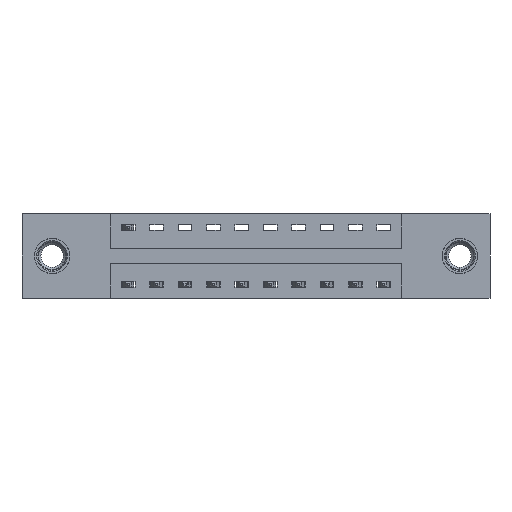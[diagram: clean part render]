
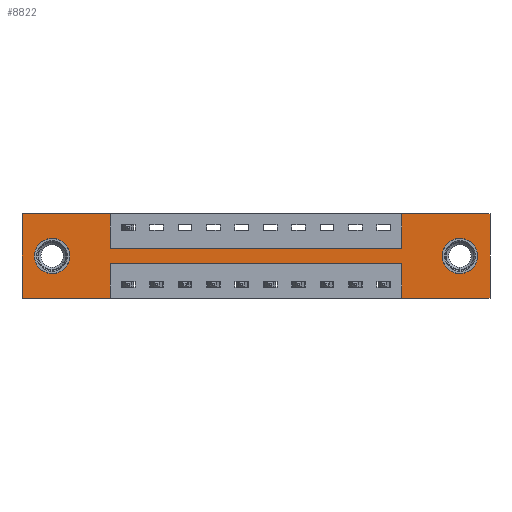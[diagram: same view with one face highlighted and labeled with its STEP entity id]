
A CAD part, front view. The second image highlights one B-rep face of the part: STEP entity #8822.
In plain terms, the highlighted planar face has unit normal (0, -1, 0).
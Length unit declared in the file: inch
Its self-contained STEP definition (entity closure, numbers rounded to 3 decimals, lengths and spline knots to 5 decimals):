
#252 = DIRECTION ( 'NONE',  ( 1., 0., 0. ) ) ;
#266 = VECTOR ( 'NONE', #3490, 39.37008 ) ;
#340 = AXIS2_PLACEMENT_3D ( 'NONE', #9653, #4228, #10537 ) ;
#367 = EDGE_CURVE ( 'NONE', #6139, #8540, #7498, .T. ) ;
#374 = LINE ( 'NONE', #8942, #7328 ) ;
#903 = CARTESIAN_POINT ( 'NONE',  ( 0., 0., 0. ) ) ;
#972 = CARTESIAN_POINT ( 'NONE',  ( 1.9275, 0., -0.185 ) ) ;
#976 = DIRECTION ( 'NONE',  ( -1., 0., 0. ) ) ;
#1192 = CARTESIAN_POINT ( 'NONE',  ( 1.9275, 0., -0.107 ) ) ;
#1198 = CARTESIAN_POINT ( 'NONE',  ( 1.6725, 0., -0.22 ) ) ;
#1221 = LINE ( 'NONE', #7119, #10551 ) ;
#1302 = CARTESIAN_POINT ( 'NONE',  ( 0., 0., 0. ) ) ;
#1346 = EDGE_CURVE ( 'NONE', #4024, #10152, #8497, .T. ) ;
#1392 = ORIENTED_EDGE ( 'NONE', *, *, #9641, .T. ) ;
#1459 = DIRECTION ( 'NONE',  ( -1., 0., 0. ) ) ;
#1496 = VECTOR ( 'NONE', #4390, 39.37008 ) ;
#1803 = ORIENTED_EDGE ( 'NONE', *, *, #7420, .T. ) ;
#1823 = EDGE_CURVE ( 'NONE', #10026, #1853, #6483, .T. ) ;
#1853 = VERTEX_POINT ( 'NONE', #1192 ) ;
#1889 = DIRECTION ( 'NONE',  ( 0., 0., -1. ) ) ;
#2069 = CARTESIAN_POINT ( 'NONE',  ( 1.9275, 0., -0.185 ) ) ;
#2090 = CARTESIAN_POINT ( 'NONE',  ( 1.6725, 0., -0.37 ) ) ;
#2194 = EDGE_LOOP ( 'NONE', ( #1803, #1392 ) ) ;
#2196 = DIRECTION ( 'NONE',  ( 1., 0., 0. ) ) ;
#2209 = PLANE ( 'NONE',  #7696 ) ;
#2290 = VECTOR ( 'NONE', #5743, 39.37008 ) ;
#2318 = LINE ( 'NONE', #3157, #11659 ) ;
#2573 = CARTESIAN_POINT ( 'NONE',  ( 0.3875, 0., 0. ) ) ;
#2576 = LINE ( 'NONE', #2090, #2290 ) ;
#2619 = DIRECTION ( 'NONE',  ( 0., 0., 1. ) ) ;
#2634 = ORIENTED_EDGE ( 'NONE', *, *, #9191, .T. ) ;
#2656 = ORIENTED_EDGE ( 'NONE', *, *, #367, .F. ) ;
#2724 = VECTOR ( 'NONE', #976, 39.37008 ) ;
#2778 = ORIENTED_EDGE ( 'NONE', *, *, #4403, .F. ) ;
#2842 = DIRECTION ( 'NONE',  ( 0., 1., 0. ) ) ;
#2978 = DIRECTION ( 'NONE',  ( 0., 0., -1. ) ) ;
#3028 = EDGE_LOOP ( 'NONE', ( #2634, #3465 ) ) ;
#3130 = DIRECTION ( 'NONE',  ( 0., -1., 0. ) ) ;
#3157 = CARTESIAN_POINT ( 'NONE',  ( 0., 0., -0.37 ) ) ;
#3262 = CARTESIAN_POINT ( 'NONE',  ( 1.6725, 0., -0.37 ) ) ;
#3268 = EDGE_CURVE ( 'NONE', #8540, #5853, #4088, .T. ) ;
#3384 = FACE_BOUND ( 'NONE', #2194, .T. ) ;
#3427 = CIRCLE ( 'NONE', #11123, 0.078 ) ;
#3465 = ORIENTED_EDGE ( 'NONE', *, *, #1823, .T. ) ;
#3490 = DIRECTION ( 'NONE',  ( 0., 0., -1. ) ) ;
#3493 = DIRECTION ( 'NONE',  ( 0., 0., 1. ) ) ;
#3627 = ORIENTED_EDGE ( 'NONE', *, *, #6941, .F. ) ;
#3734 = LINE ( 'NONE', #6914, #8263 ) ;
#3887 = LINE ( 'NONE', #9819, #1496 ) ;
#3912 = ORIENTED_EDGE ( 'NONE', *, *, #7568, .F. ) ;
#3925 = DIRECTION ( 'NONE',  ( 1., 0., 0. ) ) ;
#3987 = VERTEX_POINT ( 'NONE', #1198 ) ;
#4024 = VERTEX_POINT ( 'NONE', #7601 ) ;
#4077 = ORIENTED_EDGE ( 'NONE', *, *, #1346, .F. ) ;
#4088 = LINE ( 'NONE', #11111, #10723 ) ;
#4228 = DIRECTION ( 'NONE',  ( 0., 1., 0. ) ) ;
#4321 = VERTEX_POINT ( 'NONE', #7963 ) ;
#4349 = ORIENTED_EDGE ( 'NONE', *, *, #7541, .F. ) ;
#4390 = DIRECTION ( 'NONE',  ( 0., 0., -1. ) ) ;
#4403 = EDGE_CURVE ( 'NONE', #5853, #4321, #1221, .T. ) ;
#4492 = VERTEX_POINT ( 'NONE', #903 ) ;
#4601 = ORIENTED_EDGE ( 'NONE', *, *, #11670, .F. ) ;
#4833 = CIRCLE ( 'NONE', #7230, 0.078 ) ;
#5074 = AXIS2_PLACEMENT_3D ( 'NONE', #2069, #8426, #2978 ) ;
#5113 = LINE ( 'NONE', #6392, #2724 ) ;
#5253 = EDGE_CURVE ( 'NONE', #5287, #4024, #3887, .T. ) ;
#5287 = VERTEX_POINT ( 'NONE', #8041 ) ;
#5443 = CARTESIAN_POINT ( 'NONE',  ( 0.3875, 0., -0.15 ) ) ;
#5524 = CARTESIAN_POINT ( 'NONE',  ( 0.1325, 0., -0.263 ) ) ;
#5576 = CARTESIAN_POINT ( 'NONE',  ( 0.3875, 0., 0. ) ) ;
#5631 = EDGE_CURVE ( 'NONE', #10966, #6273, #2318, .T. ) ;
#5743 = DIRECTION ( 'NONE',  ( 0., 0., 1. ) ) ;
#5853 = VERTEX_POINT ( 'NONE', #7983 ) ;
#5865 = DIRECTION ( 'NONE',  ( -1., 0., 0. ) ) ;
#6052 = VECTOR ( 'NONE', #1459, 39.37008 ) ;
#6139 = VERTEX_POINT ( 'NONE', #5576 ) ;
#6273 = VERTEX_POINT ( 'NONE', #8519 ) ;
#6392 = CARTESIAN_POINT ( 'NONE',  ( 0.3875, 0., -0.22 ) ) ;
#6483 = CIRCLE ( 'NONE', #5074, 0.078 ) ;
#6914 = CARTESIAN_POINT ( 'NONE',  ( 0.3875, 0., -0.37 ) ) ;
#6941 = EDGE_CURVE ( 'NONE', #4321, #5287, #8425, .T. ) ;
#7119 = CARTESIAN_POINT ( 'NONE',  ( 1.6725, 0., 0. ) ) ;
#7153 = EDGE_CURVE ( 'NONE', #8580, #10966, #3734, .T. ) ;
#7196 = ORIENTED_EDGE ( 'NONE', *, *, #7401, .F. ) ;
#7230 = AXIS2_PLACEMENT_3D ( 'NONE', #8281, #2842, #9211 ) ;
#7307 = DIRECTION ( 'NONE',  ( 0., 1., 0. ) ) ;
#7328 = VECTOR ( 'NONE', #3493, 39.37008 ) ;
#7401 = EDGE_CURVE ( 'NONE', #3987, #8580, #5113, .T. ) ;
#7420 = EDGE_CURVE ( 'NONE', #8113, #10554, #4833, .T. ) ;
#7498 = LINE ( 'NONE', #2573, #266 ) ;
#7541 = EDGE_CURVE ( 'NONE', #10152, #3987, #2576, .T. ) ;
#7568 = EDGE_CURVE ( 'NONE', #4492, #6139, #9257, .T. ) ;
#7601 = CARTESIAN_POINT ( 'NONE',  ( 2.06, 0., -0.37 ) ) ;
#7696 = AXIS2_PLACEMENT_3D ( 'NONE', #8582, #3130, #9472 ) ;
#7728 = CARTESIAN_POINT ( 'NONE',  ( 0., 0., -0.37 ) ) ;
#7916 = FACE_OUTER_BOUND ( 'NONE', #8003, .T. ) ;
#7963 = CARTESIAN_POINT ( 'NONE',  ( 1.6725, 0., 0. ) ) ;
#7983 = CARTESIAN_POINT ( 'NONE',  ( 1.6725, 0., -0.15 ) ) ;
#8003 = EDGE_LOOP ( 'NONE', ( #9877, #7196, #4349, #4077, #8021, #3627, #2778, #9172, #2656, #3912, #4601, #11711 ) ) ;
#8021 = ORIENTED_EDGE ( 'NONE', *, *, #5253, .F. ) ;
#8041 = CARTESIAN_POINT ( 'NONE',  ( 2.06, 0., 0. ) ) ;
#8113 = VERTEX_POINT ( 'NONE', #9300 ) ;
#8263 = VECTOR ( 'NONE', #8701, 39.37008 ) ;
#8281 = CARTESIAN_POINT ( 'NONE',  ( 0.1325, 0., -0.185 ) ) ;
#8425 = LINE ( 'NONE', #11168, #10231 ) ;
#8426 = DIRECTION ( 'NONE',  ( 0., 1., 0. ) ) ;
#8497 = LINE ( 'NONE', #7728, #6052 ) ;
#8519 = CARTESIAN_POINT ( 'NONE',  ( 0., 0., -0.37 ) ) ;
#8540 = VERTEX_POINT ( 'NONE', #5443 ) ;
#8580 = VERTEX_POINT ( 'NONE', #10012 ) ;
#8582 = CARTESIAN_POINT ( 'NONE',  ( 0., 0., -0.37 ) ) ;
#8701 = DIRECTION ( 'NONE',  ( 0., 0., -1. ) ) ;
#8822 = ADVANCED_FACE ( 'NONE', ( #10311, #3384, #7916 ), #2209, .T. ) ;
#8942 = CARTESIAN_POINT ( 'NONE',  ( 0., 0., 0. ) ) ;
#9172 = ORIENTED_EDGE ( 'NONE', *, *, #3268, .F. ) ;
#9191 = EDGE_CURVE ( 'NONE', #1853, #10026, #3427, .T. ) ;
#9211 = DIRECTION ( 'NONE',  ( 0., 0., 1. ) ) ;
#9257 = LINE ( 'NONE', #1302, #11347 ) ;
#9300 = CARTESIAN_POINT ( 'NONE',  ( 0.1325, 0., -0.107 ) ) ;
#9472 = DIRECTION ( 'NONE',  ( 0., 0., -1. ) ) ;
#9610 = CARTESIAN_POINT ( 'NONE',  ( 0.3875, 0., -0.37 ) ) ;
#9641 = EDGE_CURVE ( 'NONE', #10554, #8113, #10909, .T. ) ;
#9653 = CARTESIAN_POINT ( 'NONE',  ( 0.1325, 0., -0.185 ) ) ;
#9819 = CARTESIAN_POINT ( 'NONE',  ( 2.06, 0., 0. ) ) ;
#9877 = ORIENTED_EDGE ( 'NONE', *, *, #7153, .F. ) ;
#10012 = CARTESIAN_POINT ( 'NONE',  ( 0.3875, 0., -0.22 ) ) ;
#10026 = VERTEX_POINT ( 'NONE', #10261 ) ;
#10152 = VERTEX_POINT ( 'NONE', #3262 ) ;
#10231 = VECTOR ( 'NONE', #3925, 39.37008 ) ;
#10261 = CARTESIAN_POINT ( 'NONE',  ( 1.9275, 0., -0.263 ) ) ;
#10311 = FACE_BOUND ( 'NONE', #3028, .T. ) ;
#10537 = DIRECTION ( 'NONE',  ( 0., 0., 1. ) ) ;
#10551 = VECTOR ( 'NONE', #2619, 39.37008 ) ;
#10554 = VERTEX_POINT ( 'NONE', #5524 ) ;
#10723 = VECTOR ( 'NONE', #252, 39.37008 ) ;
#10909 = CIRCLE ( 'NONE', #340, 0.078 ) ;
#10966 = VERTEX_POINT ( 'NONE', #9610 ) ;
#11111 = CARTESIAN_POINT ( 'NONE',  ( 0.3875, 0., -0.15 ) ) ;
#11123 = AXIS2_PLACEMENT_3D ( 'NONE', #972, #7307, #1889 ) ;
#11168 = CARTESIAN_POINT ( 'NONE',  ( 0., 0., 0. ) ) ;
#11347 = VECTOR ( 'NONE', #2196, 39.37008 ) ;
#11659 = VECTOR ( 'NONE', #5865, 39.37008 ) ;
#11670 = EDGE_CURVE ( 'NONE', #6273, #4492, #374, .T. ) ;
#11711 = ORIENTED_EDGE ( 'NONE', *, *, #5631, .F. ) ;
